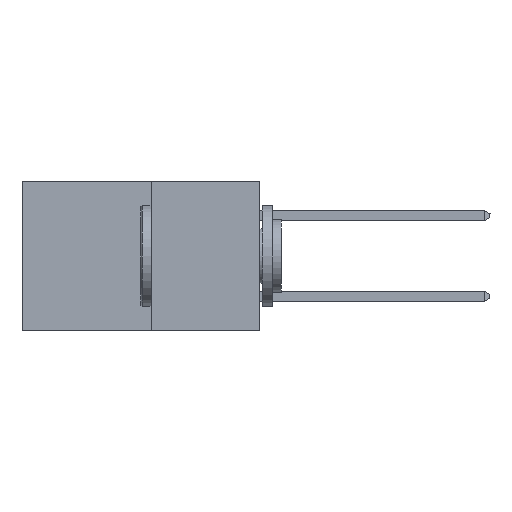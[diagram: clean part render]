
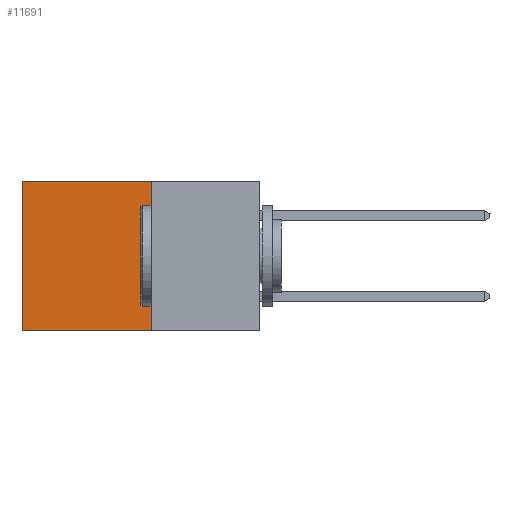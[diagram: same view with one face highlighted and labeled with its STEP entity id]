
A CAD part, left-side view. The second image highlights one B-rep face of the part: STEP entity #11691.
In plain terms, the highlighted planar face has unit normal (-1, 0, 0).
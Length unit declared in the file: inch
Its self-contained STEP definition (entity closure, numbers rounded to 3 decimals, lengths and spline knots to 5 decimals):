
#145 = LINE ( 'NONE', #9670, #5617 ) ;
#257 = VECTOR ( 'NONE', #9768, 39.37008 ) ;
#661 = EDGE_CURVE ( 'NONE', #4732, #9206, #145, .T. ) ;
#1411 = EDGE_LOOP ( 'NONE', ( #4983, #10899, #3400, #12246 ) ) ;
#2208 = CARTESIAN_POINT ( 'NONE',  ( 0.277, 0.27, -0.37 ) ) ;
#2988 = LINE ( 'NONE', #4617, #257 ) ;
#3241 = DIRECTION ( 'NONE',  ( 0., 0., -1. ) ) ;
#3400 = ORIENTED_EDGE ( 'NONE', *, *, #11980, .F. ) ;
#3788 = CARTESIAN_POINT ( 'NONE',  ( 0.277, 0.27, -0.37 ) ) ;
#3827 = DIRECTION ( 'NONE',  ( 1., 0., 0. ) ) ;
#4521 = LINE ( 'NONE', #2208, #12047 ) ;
#4617 = CARTESIAN_POINT ( 'NONE',  ( 0.277, 0.27, -0.37 ) ) ;
#4732 = VERTEX_POINT ( 'NONE', #8807 ) ;
#4780 = AXIS2_PLACEMENT_3D ( 'NONE', #3788, #3827, #10977 ) ;
#4852 = VERTEX_POINT ( 'NONE', #8303 ) ;
#4983 = ORIENTED_EDGE ( 'NONE', *, *, #661, .T. ) ;
#5617 = VECTOR ( 'NONE', #12521, 39.37008 ) ;
#6499 = EDGE_CURVE ( 'NONE', #10089, #4732, #11698, .T. ) ;
#6912 = CARTESIAN_POINT ( 'NONE',  ( 0.277, 0.59, -0.37 ) ) ;
#8303 = CARTESIAN_POINT ( 'NONE',  ( 0.277, 0.27, -0.37 ) ) ;
#8807 = CARTESIAN_POINT ( 'NONE',  ( 0.277, 0.59, 0. ) ) ;
#9009 = VECTOR ( 'NONE', #9816, 39.37008 ) ;
#9096 = EDGE_CURVE ( 'NONE', #4852, #9206, #2988, .T. ) ;
#9206 = VERTEX_POINT ( 'NONE', #6912 ) ;
#9670 = CARTESIAN_POINT ( 'NONE',  ( 0.277, 0.59, -0.37 ) ) ;
#9768 = DIRECTION ( 'NONE',  ( 0., 1., 0. ) ) ;
#9816 = DIRECTION ( 'NONE',  ( 0., 1., 0. ) ) ;
#9958 = PLANE ( 'NONE',  #4780 ) ;
#10034 = CARTESIAN_POINT ( 'NONE',  ( 0.277, 0.27, 0. ) ) ;
#10089 = VERTEX_POINT ( 'NONE', #12229 ) ;
#10899 = ORIENTED_EDGE ( 'NONE', *, *, #9096, .F. ) ;
#10977 = DIRECTION ( 'NONE',  ( 0., 0., -1. ) ) ;
#11691 = ADVANCED_FACE ( 'NONE', ( #12834 ), #9958, .F. ) ;
#11698 = LINE ( 'NONE', #10034, #9009 ) ;
#11980 = EDGE_CURVE ( 'NONE', #10089, #4852, #4521, .T. ) ;
#12047 = VECTOR ( 'NONE', #3241, 39.37008 ) ;
#12229 = CARTESIAN_POINT ( 'NONE',  ( 0.277, 0.27, 0. ) ) ;
#12246 = ORIENTED_EDGE ( 'NONE', *, *, #6499, .T. ) ;
#12521 = DIRECTION ( 'NONE',  ( 0., 0., -1. ) ) ;
#12834 = FACE_OUTER_BOUND ( 'NONE', #1411, .T. ) ;
